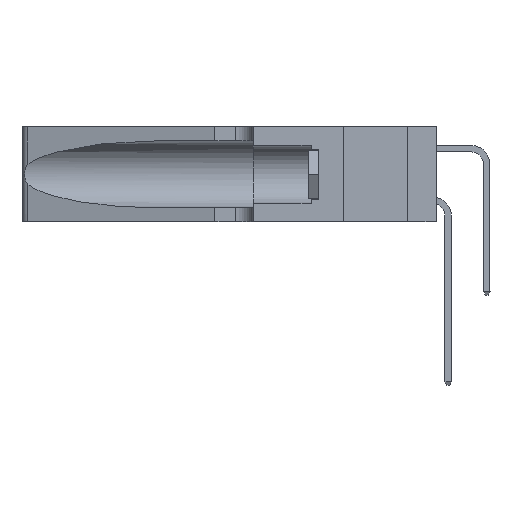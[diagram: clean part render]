
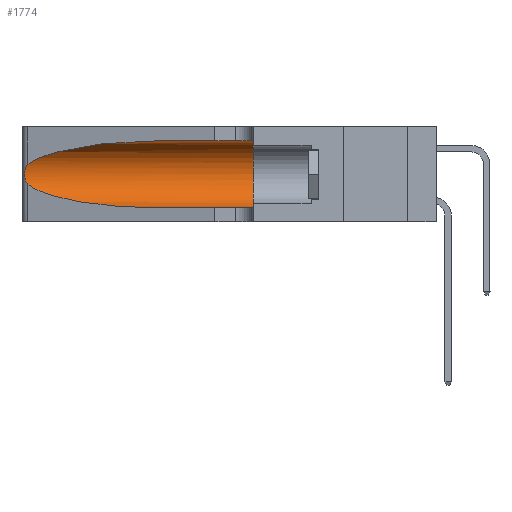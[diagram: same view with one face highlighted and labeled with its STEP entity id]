
A CAD part, left-side view. The second image highlights one B-rep face of the part: STEP entity #1774.
In plain terms, the highlighted cylindrical face has radius 3.308 mm (diameter 6.617 mm), a partial arc.
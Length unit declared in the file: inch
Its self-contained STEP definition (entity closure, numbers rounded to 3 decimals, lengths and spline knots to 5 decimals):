
#210 =( BOUNDED_CURVE ( )  B_SPLINE_CURVE ( 3, ( #504, #2576, #16741, #4711 ),
 .UNSPECIFIED., .F., .F. ) 
 B_SPLINE_CURVE_WITH_KNOTS ( ( 4, 4 ),
 ( 1.5708, 2.84003 ),
 .UNSPECIFIED. ) 
 CURVE ( )  GEOMETRIC_REPRESENTATION_ITEM ( )  RATIONAL_B_SPLINE_CURVE ( ( 1., 0.87, 0.87, 1. ) ) 
 REPRESENTATION_ITEM ( '' )  );
#504 = CARTESIAN_POINT ( 'NONE',  ( 0.1305, 0.72297, 0.31525 ) ) ;
#603 = ORIENTED_EDGE ( 'NONE', *, *, #19451, .T. ) ;
#657 = EDGE_LOOP ( 'NONE', ( #603, #24400, #16442, #20125, #17404, #15865 ) ) ;
#1167 =( BOUNDED_CURVE ( )  B_SPLINE_CURVE ( 3, ( #18670, #4669, #20633, #8761 ),
 .UNSPECIFIED., .F., .F. ) 
 B_SPLINE_CURVE_WITH_KNOTS ( ( 4, 4 ),
 ( 3.44316, 4.71239 ),
 .UNSPECIFIED. ) 
 CURVE ( )  GEOMETRIC_REPRESENTATION_ITEM ( )  RATIONAL_B_SPLINE_CURVE ( ( 1., 0.87, 0.87, 1. ) ) 
 REPRESENTATION_ITEM ( '' )  );
#1543 = EDGE_CURVE ( 'NONE', #16999, #7786, #11923, .T. ) ;
#1641 = CARTESIAN_POINT ( 'NONE',  ( 0.1305, 1.61858, 0.31525 ) ) ;
#1774 = ADVANCED_FACE ( 'NONE', ( #3668 ), #13150, .F. ) ;
#1976 = CARTESIAN_POINT ( 'NONE',  ( 0.25787, 1.23484, 0.2124 ) ) ;
#2576 = CARTESIAN_POINT ( 'NONE',  ( 0.18966, 0.96281, 0.31525 ) ) ;
#3166 = B_SPLINE_CURVE_WITH_KNOTS ( 'NONE', 3,
 ( #25870, #5937, #6105, #1976, #16171, #4109, #18145, #6194, #20112, #8229, #22106, #10214, #24041, #12224 ),
 .UNSPECIFIED., .F., .F.,
 ( 4, 2, 2, 2, 2, 2, 4 ),
 ( 0., 0.00027, 0.00053, 0.00107, 0.0016, 0.00187, 0.00214 ),
 .UNSPECIFIED. ) ;
#3269 = VECTOR ( 'NONE', #9899, 39.37008 ) ;
#3586 = VERTEX_POINT ( 'NONE', #11933 ) ;
#3668 = FACE_OUTER_BOUND ( 'NONE', #657, .T. ) ;
#3945 = LINE ( 'NONE', #1641, #3269 ) ;
#4109 = CARTESIAN_POINT ( 'NONE',  ( 0.26018, 1.23835, 0.19895 ) ) ;
#4455 = EDGE_CURVE ( 'NONE', #3586, #7786, #17734, .T. ) ;
#4505 = VERTEX_POINT ( 'NONE', #15050 ) ;
#4669 = CARTESIAN_POINT ( 'NONE',  ( 0.2373, 1.15595, 0.08982 ) ) ;
#4711 = CARTESIAN_POINT ( 'NONE',  ( 0.25487, 1.22718, 0.22369 ) ) ;
#5937 = CARTESIAN_POINT ( 'NONE',  ( 0.25555, 1.22994, 0.2215 ) ) ;
#6105 = CARTESIAN_POINT ( 'NONE',  ( 0.25639, 1.23184, 0.21858 ) ) ;
#6183 = CARTESIAN_POINT ( 'NONE',  ( 0.1305, 0.35, 0.31525 ) ) ;
#6194 = CARTESIAN_POINT ( 'NONE',  ( 0.26075, 1.23896, 0.178 ) ) ;
#7004 = CARTESIAN_POINT ( 'NONE',  ( 0.25487, 1.22718, 0.14631 ) ) ;
#7508 = EDGE_CURVE ( 'NONE', #22047, #21540, #3166, .T. ) ;
#7786 = VERTEX_POINT ( 'NONE', #18894 ) ;
#8229 = CARTESIAN_POINT ( 'NONE',  ( 0.25856, 1.23593, 0.16098 ) ) ;
#8761 = CARTESIAN_POINT ( 'NONE',  ( 0.1305, 0.72297, 0.05475 ) ) ;
#9899 = DIRECTION ( 'NONE',  ( 0., -1., 0. ) ) ;
#10214 = CARTESIAN_POINT ( 'NONE',  ( 0.25639, 1.23186, 0.15144 ) ) ;
#10654 = CARTESIAN_POINT ( 'NONE',  ( 0.1305, 0.35, 0.185 ) ) ;
#11923 = CIRCLE ( 'NONE', #23264, 0.13025 ) ;
#11933 = CARTESIAN_POINT ( 'NONE',  ( 0.1305, 0.72297, 0.05475 ) ) ;
#12224 = CARTESIAN_POINT ( 'NONE',  ( 0.25487, 1.22718, 0.14631 ) ) ;
#12439 = VECTOR ( 'NONE', #12948, 39.37008 ) ;
#12948 = DIRECTION ( 'NONE',  ( 0., -1., 0. ) ) ;
#13150 = CYLINDRICAL_SURFACE ( 'NONE', #24074, 0.13025 ) ;
#15050 = CARTESIAN_POINT ( 'NONE',  ( 0.1305, 0.72297, 0.31525 ) ) ;
#15865 = ORIENTED_EDGE ( 'NONE', *, *, #22962, .F. ) ;
#16171 = CARTESIAN_POINT ( 'NONE',  ( 0.25854, 1.2359, 0.20912 ) ) ;
#16442 = ORIENTED_EDGE ( 'NONE', *, *, #16498, .T. ) ;
#16498 = EDGE_CURVE ( 'NONE', #21540, #3586, #1167, .T. ) ;
#16741 = CARTESIAN_POINT ( 'NONE',  ( 0.2373, 1.15595, 0.28018 ) ) ;
#16999 = VERTEX_POINT ( 'NONE', #6183 ) ;
#17404 = ORIENTED_EDGE ( 'NONE', *, *, #1543, .F. ) ;
#17734 = LINE ( 'NONE', #20819, #12439 ) ;
#18145 = CARTESIAN_POINT ( 'NONE',  ( 0.26075, 1.23896, 0.19203 ) ) ;
#18670 = CARTESIAN_POINT ( 'NONE',  ( 0.25487, 1.22718, 0.14631 ) ) ;
#18894 = CARTESIAN_POINT ( 'NONE',  ( 0.1305, 0.35, 0.05475 ) ) ;
#19451 = EDGE_CURVE ( 'NONE', #4505, #22047, #210, .T. ) ;
#19782 = DIRECTION ( 'NONE',  ( 0., 0., 1. ) ) ;
#19789 = DIRECTION ( 'NONE',  ( 0., 1., 0. ) ) ;
#20112 = CARTESIAN_POINT ( 'NONE',  ( 0.26017, 1.23833, 0.17102 ) ) ;
#20125 = ORIENTED_EDGE ( 'NONE', *, *, #4455, .T. ) ;
#20633 = CARTESIAN_POINT ( 'NONE',  ( 0.18966, 0.96281, 0.05475 ) ) ;
#20749 = CARTESIAN_POINT ( 'NONE',  ( 0.1305, 1.61858, 0.185 ) ) ;
#20810 = DIRECTION ( 'NONE',  ( 0., 0., -1. ) ) ;
#20819 = CARTESIAN_POINT ( 'NONE',  ( 0.1305, 1.61858, 0.05475 ) ) ;
#21540 = VERTEX_POINT ( 'NONE', #7004 ) ;
#22047 = VERTEX_POINT ( 'NONE', #24859 ) ;
#22106 = CARTESIAN_POINT ( 'NONE',  ( 0.25789, 1.23486, 0.15765 ) ) ;
#22865 = DIRECTION ( 'NONE',  ( 0., -1., 0. ) ) ;
#22962 = EDGE_CURVE ( 'NONE', #4505, #16999, #3945, .T. ) ;
#23264 = AXIS2_PLACEMENT_3D ( 'NONE', #10654, #19789, #19782 ) ;
#24041 = CARTESIAN_POINT ( 'NONE',  ( 0.25555, 1.22993, 0.14849 ) ) ;
#24074 = AXIS2_PLACEMENT_3D ( 'NONE', #20749, #22865, #20810 ) ;
#24400 = ORIENTED_EDGE ( 'NONE', *, *, #7508, .T. ) ;
#24859 = CARTESIAN_POINT ( 'NONE',  ( 0.25487, 1.22718, 0.22369 ) ) ;
#25870 = CARTESIAN_POINT ( 'NONE',  ( 0.25487, 1.22718, 0.22369 ) ) ;
